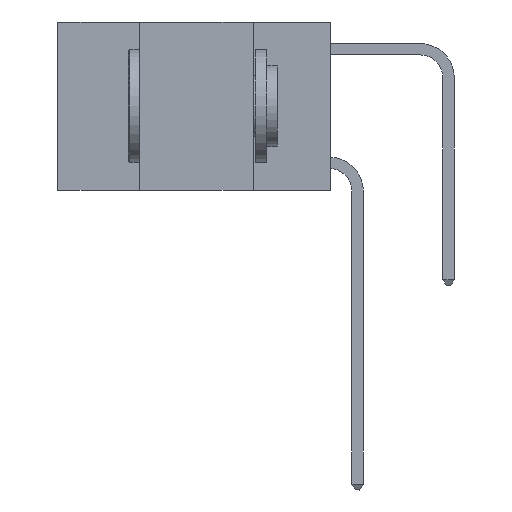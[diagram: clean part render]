
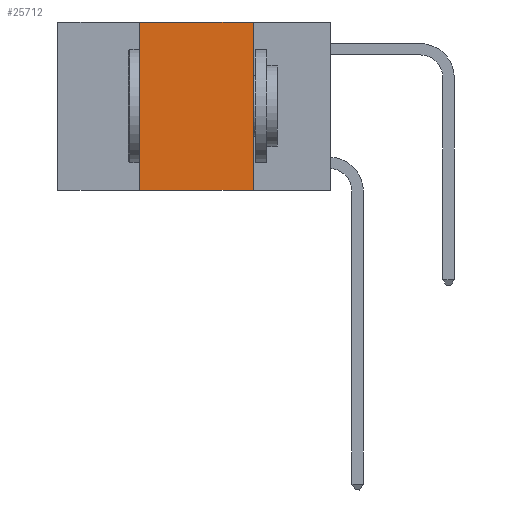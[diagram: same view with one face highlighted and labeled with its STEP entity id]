
A CAD part, left-side view. The second image highlights one B-rep face of the part: STEP entity #25712.
In plain terms, the highlighted planar face has unit normal (-1, 0, 0).
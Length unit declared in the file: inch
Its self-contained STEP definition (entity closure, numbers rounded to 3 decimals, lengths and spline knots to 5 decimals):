
#477 = DIRECTION ( 'NONE',  ( 0., 0., -1. ) ) ;
#1207 = LINE ( 'NONE', #3072, #19736 ) ;
#2434 = PLANE ( 'NONE',  #18387 ) ;
#3072 = CARTESIAN_POINT ( 'NONE',  ( 0., 0.42, 0. ) ) ;
#4289 = LINE ( 'NONE', #10401, #9637 ) ;
#4584 = EDGE_CURVE ( 'NONE', #6662, #8786, #16036, .T. ) ;
#5320 = DIRECTION ( 'NONE',  ( 0., 0., -1. ) ) ;
#5920 = CARTESIAN_POINT ( 'NONE',  ( 0., 0.42, -0.37 ) ) ;
#6220 = DIRECTION ( 'NONE',  ( 0., -1., 0. ) ) ;
#6587 = ORIENTED_EDGE ( 'NONE', *, *, #4584, .T. ) ;
#6662 = VERTEX_POINT ( 'NONE', #5920 ) ;
#7287 = CARTESIAN_POINT ( 'NONE',  ( 0., 0.17, 0. ) ) ;
#8441 = CARTESIAN_POINT ( 'NONE',  ( 0., 0.6, -0.37 ) ) ;
#8511 = LINE ( 'NONE', #7287, #15922 ) ;
#8786 = VERTEX_POINT ( 'NONE', #11618 ) ;
#9637 = VECTOR ( 'NONE', #6220, 39.37008 ) ;
#10038 = VERTEX_POINT ( 'NONE', #12937 ) ;
#10401 = CARTESIAN_POINT ( 'NONE',  ( 0., 0.6, 0. ) ) ;
#10404 = CARTESIAN_POINT ( 'NONE',  ( 0., 0.6, 0. ) ) ;
#10924 = FACE_OUTER_BOUND ( 'NONE', #18083, .T. ) ;
#11618 = CARTESIAN_POINT ( 'NONE',  ( 0., 0.17, -0.37 ) ) ;
#12708 = ORIENTED_EDGE ( 'NONE', *, *, #22666, .F. ) ;
#12937 = CARTESIAN_POINT ( 'NONE',  ( 0., 0.42, 0. ) ) ;
#13124 = DIRECTION ( 'NONE',  ( 0., 0., 1. ) ) ;
#15804 = VECTOR ( 'NONE', #16416, 39.37008 ) ;
#15922 = VECTOR ( 'NONE', #5320, 39.37008 ) ;
#16036 = LINE ( 'NONE', #8441, #15804 ) ;
#16416 = DIRECTION ( 'NONE',  ( 0., -1., 0. ) ) ;
#16848 = CARTESIAN_POINT ( 'NONE',  ( 0., 0.17, 0. ) ) ;
#18083 = EDGE_LOOP ( 'NONE', ( #19195, #25628, #12708, #6587 ) ) ;
#18385 = DIRECTION ( 'NONE',  ( 1., 0., 0. ) ) ;
#18387 = AXIS2_PLACEMENT_3D ( 'NONE', #10404, #18385, #477 ) ;
#19195 = ORIENTED_EDGE ( 'NONE', *, *, #19395, .F. ) ;
#19395 = EDGE_CURVE ( 'NONE', #25186, #8786, #8511, .T. ) ;
#19677 = EDGE_CURVE ( 'NONE', #10038, #25186, #4289, .T. ) ;
#19736 = VECTOR ( 'NONE', #13124, 39.37008 ) ;
#22666 = EDGE_CURVE ( 'NONE', #6662, #10038, #1207, .T. ) ;
#25186 = VERTEX_POINT ( 'NONE', #16848 ) ;
#25628 = ORIENTED_EDGE ( 'NONE', *, *, #19677, .F. ) ;
#25712 = ADVANCED_FACE ( 'NONE', ( #10924 ), #2434, .F. ) ;
